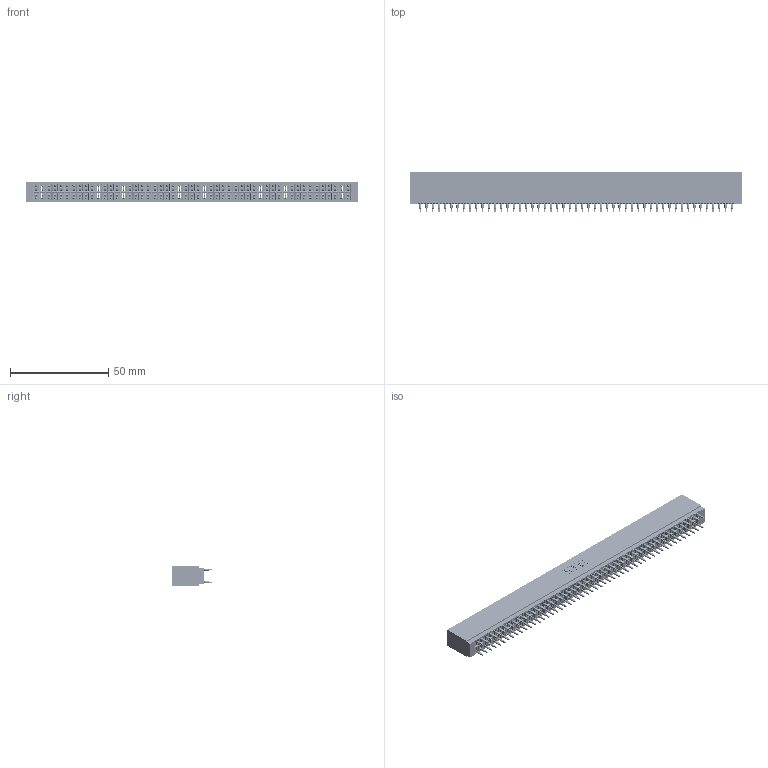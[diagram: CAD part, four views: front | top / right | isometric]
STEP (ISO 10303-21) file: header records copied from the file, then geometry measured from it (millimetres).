
FILE_DESCRIPTION (( 'STEP AP203' ), '1' );
FILE_NAME ('746-102-560-201.STEP', '2026-03-04T23:01:20', ( '' ), ( '' ), 'SwSTEP 2.0', 'SolidWorks 2023', '' );
FILE_SCHEMA (( 'CONFIG_CONTROL_DESIGN' ));
Length unit declared in the file: millimetre
Products named in the file (3): 746-292-001_560; 746 Part_.515 Slot Depth - 01; 746-102-560-201
Assembly tree (103 placements, depth 2):
  746-102-560-201
    746 Part_.515 Slot Depth - 01
    746-292-001_560  x102
Bounding box: 169.16 x 20.82 x 9.91 mm (x, y, z)
Volume: 18428 mm3; surface area: 31434.5 mm2
Topology: 103 solids, 103 shells, 9736 faces, 27089 edges, 17362 vertices
Faces by surface type: plane 4849, cylinder 2235, bspline 2040, torus 612
Entity records: 77618 total; most frequent: CARTESIAN_POINT 15349, ORIENTED_EDGE 13374, DIRECTION 11157, EDGE_CURVE 6687, LINE 5985, VECTOR 5985, VERTEX_POINT 4434, AXIS2_PLACEMENT_3D 2586
